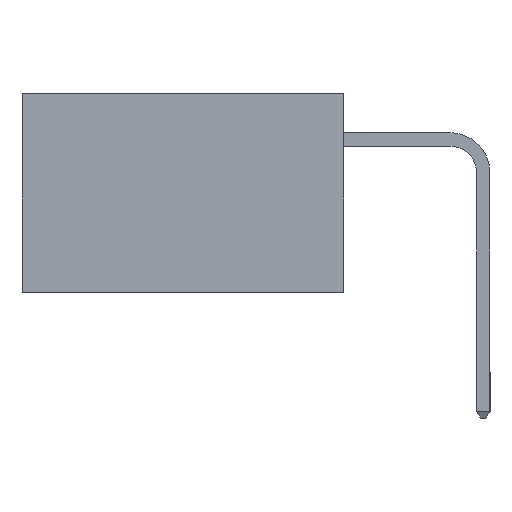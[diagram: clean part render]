
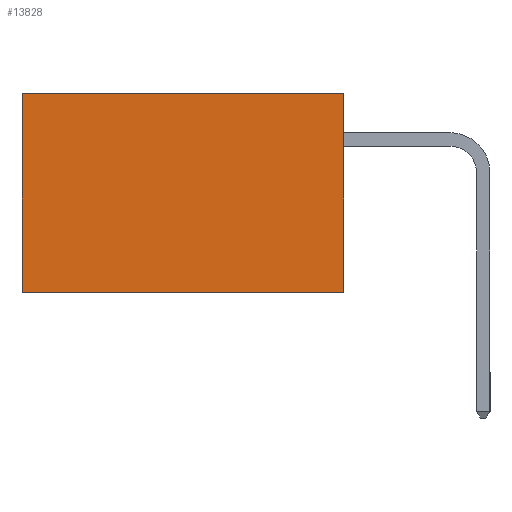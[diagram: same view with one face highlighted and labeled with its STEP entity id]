
A CAD part, left-side view. The second image highlights one B-rep face of the part: STEP entity #13828.
In plain terms, the highlighted planar face has unit normal (-1, 0, 0).
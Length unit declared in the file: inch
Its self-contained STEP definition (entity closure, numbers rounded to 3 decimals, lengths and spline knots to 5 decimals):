
#488 = FACE_OUTER_BOUND ( 'NONE', #18043, .T. ) ;
#1003 = VERTEX_POINT ( 'NONE', #12316 ) ;
#1581 = LINE ( 'NONE', #17675, #2803 ) ;
#1601 = CARTESIAN_POINT ( 'NONE',  ( 0.298, 0., 0. ) ) ;
#2139 = DIRECTION ( 'NONE',  ( 0., 0., -1. ) ) ;
#2803 = VECTOR ( 'NONE', #10033, 39.37008 ) ;
#3003 = VERTEX_POINT ( 'NONE', #1601 ) ;
#3550 = LINE ( 'NONE', #5306, #6917 ) ;
#3577 = DIRECTION ( 'NONE',  ( 1., 0., 0. ) ) ;
#4465 = DIRECTION ( 'NONE',  ( 0., 1., 0. ) ) ;
#4744 = ORIENTED_EDGE ( 'NONE', *, *, #17460, .F. ) ;
#5306 = CARTESIAN_POINT ( 'NONE',  ( 0.298, 0., 0. ) ) ;
#5713 = VERTEX_POINT ( 'NONE', #14076 ) ;
#6917 = VECTOR ( 'NONE', #16138, 39.37008 ) ;
#7262 = CARTESIAN_POINT ( 'NONE',  ( 0.298, 0., 0. ) ) ;
#7577 = EDGE_CURVE ( 'NONE', #17076, #1003, #1581, .T. ) ;
#8768 = VECTOR ( 'NONE', #4465, 39.37008 ) ;
#9787 = CARTESIAN_POINT ( 'NONE',  ( 0.298, 0., 0. ) ) ;
#10033 = DIRECTION ( 'NONE',  ( 0., 0., -1. ) ) ;
#10301 = EDGE_CURVE ( 'NONE', #3003, #5713, #3550, .T. ) ;
#11269 = ORIENTED_EDGE ( 'NONE', *, *, #7577, .T. ) ;
#12316 = CARTESIAN_POINT ( 'NONE',  ( 0.298, 0.6, -0.37 ) ) ;
#12660 = ORIENTED_EDGE ( 'NONE', *, *, #19707, .T. ) ;
#12882 = LINE ( 'NONE', #18292, #8768 ) ;
#13163 = ORIENTED_EDGE ( 'NONE', *, *, #10301, .F. ) ;
#13828 = ADVANCED_FACE ( 'NONE', ( #488 ), #17639, .F. ) ;
#14076 = CARTESIAN_POINT ( 'NONE',  ( 0.298, 0., -0.37 ) ) ;
#14470 = LINE ( 'NONE', #7262, #19505 ) ;
#16138 = DIRECTION ( 'NONE',  ( 0., 0., -1. ) ) ;
#16620 = DIRECTION ( 'NONE',  ( 0., 1., 0. ) ) ;
#17076 = VERTEX_POINT ( 'NONE', #18714 ) ;
#17203 = AXIS2_PLACEMENT_3D ( 'NONE', #9787, #3577, #2139 ) ;
#17460 = EDGE_CURVE ( 'NONE', #5713, #1003, #12882, .T. ) ;
#17639 = PLANE ( 'NONE',  #17203 ) ;
#17675 = CARTESIAN_POINT ( 'NONE',  ( 0.298, 0.6, 0. ) ) ;
#18043 = EDGE_LOOP ( 'NONE', ( #11269, #4744, #13163, #12660 ) ) ;
#18292 = CARTESIAN_POINT ( 'NONE',  ( 0.298, 0., -0.37 ) ) ;
#18714 = CARTESIAN_POINT ( 'NONE',  ( 0.298, 0.6, 0. ) ) ;
#19505 = VECTOR ( 'NONE', #16620, 39.37008 ) ;
#19707 = EDGE_CURVE ( 'NONE', #3003, #17076, #14470, .T. ) ;
